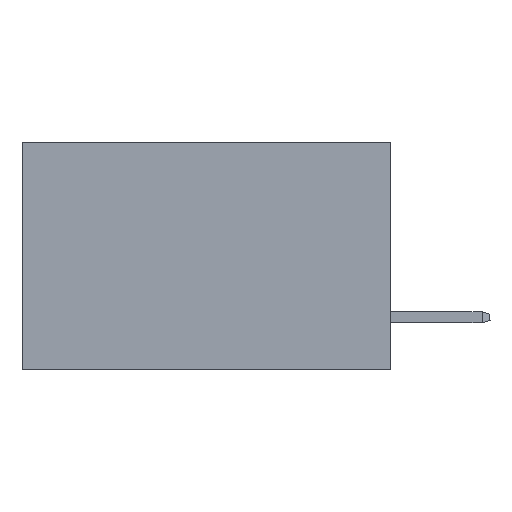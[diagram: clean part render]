
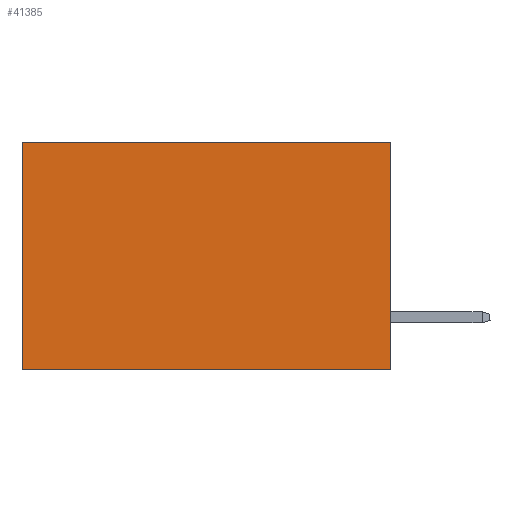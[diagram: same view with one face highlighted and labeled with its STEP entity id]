
A CAD part, left-side view. The second image highlights one B-rep face of the part: STEP entity #41385.
In plain terms, the highlighted planar face has unit normal (-1, 0, 0).
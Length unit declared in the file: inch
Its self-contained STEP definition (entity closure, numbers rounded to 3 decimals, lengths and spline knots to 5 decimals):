
#267 = FACE_OUTER_BOUND ( 'NONE', #23061, .T. ) ;
#700 = DIRECTION ( 'NONE',  ( 0., 0., -1. ) ) ;
#1668 = EDGE_CURVE ( 'NONE', #31487, #24022, #8313, .T. ) ;
#1675 = DIRECTION ( 'NONE',  ( 0., 1., 0. ) ) ;
#1988 = DIRECTION ( 'NONE',  ( 0., 0., -1. ) ) ;
#2392 = LINE ( 'NONE', #33806, #19045 ) ;
#2586 = VECTOR ( 'NONE', #1675, 39.37008 ) ;
#3644 = DIRECTION ( 'NONE',  ( 1., 0., 0. ) ) ;
#6135 = VERTEX_POINT ( 'NONE', #28070 ) ;
#6809 = VERTEX_POINT ( 'NONE', #22625 ) ;
#7586 = VECTOR ( 'NONE', #1988, 39.37008 ) ;
#8313 = LINE ( 'NONE', #14898, #2586 ) ;
#10467 = CARTESIAN_POINT ( 'NONE',  ( 0.2875, 0., 0. ) ) ;
#10606 = EDGE_CURVE ( 'NONE', #6809, #24022, #41006, .T. ) ;
#10974 = EDGE_CURVE ( 'NONE', #6135, #6809, #2392, .T. ) ;
#11029 = ORIENTED_EDGE ( 'NONE', *, *, #21004, .F. ) ;
#11759 = LINE ( 'NONE', #41739, #7586 ) ;
#14898 = CARTESIAN_POINT ( 'NONE',  ( 0.2875, 0., -0.37 ) ) ;
#16647 = CARTESIAN_POINT ( 'NONE',  ( 0.2875, 0.6, 0. ) ) ;
#17076 = CARTESIAN_POINT ( 'NONE',  ( 0.2875, 0.6, -0.37 ) ) ;
#18882 = AXIS2_PLACEMENT_3D ( 'NONE', #10467, #3644, #700 ) ;
#19045 = VECTOR ( 'NONE', #38368, 39.37008 ) ;
#20511 = PLANE ( 'NONE',  #18882 ) ;
#20531 = ORIENTED_EDGE ( 'NONE', *, *, #10606, .T. ) ;
#21004 = EDGE_CURVE ( 'NONE', #6135, #31487, #11759, .T. ) ;
#22625 = CARTESIAN_POINT ( 'NONE',  ( 0.2875, 0.6, 0. ) ) ;
#23061 = EDGE_LOOP ( 'NONE', ( #20531, #42920, #11029, #32011 ) ) ;
#24022 = VERTEX_POINT ( 'NONE', #17076 ) ;
#28070 = CARTESIAN_POINT ( 'NONE',  ( 0.2875, 0., 0. ) ) ;
#29893 = DIRECTION ( 'NONE',  ( 0., 0., -1. ) ) ;
#30009 = VECTOR ( 'NONE', #29893, 39.37008 ) ;
#31487 = VERTEX_POINT ( 'NONE', #42088 ) ;
#32011 = ORIENTED_EDGE ( 'NONE', *, *, #10974, .T. ) ;
#33806 = CARTESIAN_POINT ( 'NONE',  ( 0.2875, 0., 0. ) ) ;
#38368 = DIRECTION ( 'NONE',  ( 0., 1., 0. ) ) ;
#41006 = LINE ( 'NONE', #16647, #30009 ) ;
#41385 = ADVANCED_FACE ( 'NONE', ( #267 ), #20511, .F. ) ;
#41739 = CARTESIAN_POINT ( 'NONE',  ( 0.2875, 0., 0. ) ) ;
#42088 = CARTESIAN_POINT ( 'NONE',  ( 0.2875, 0., -0.37 ) ) ;
#42920 = ORIENTED_EDGE ( 'NONE', *, *, #1668, .F. ) ;
